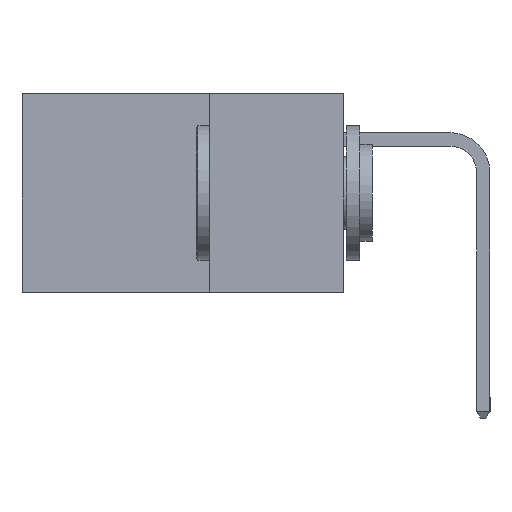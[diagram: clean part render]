
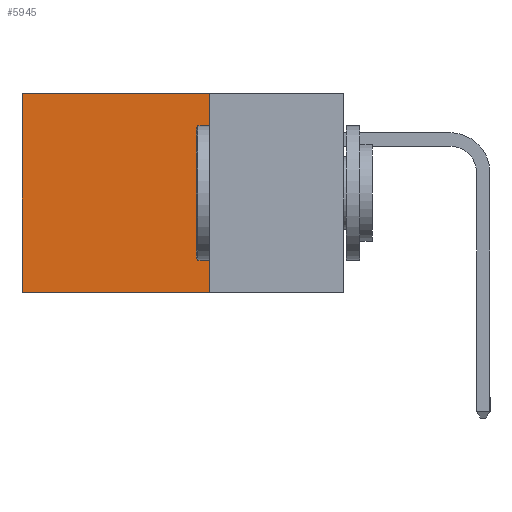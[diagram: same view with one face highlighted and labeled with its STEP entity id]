
A CAD part, left-side view. The second image highlights one B-rep face of the part: STEP entity #5945.
In plain terms, the highlighted planar face has unit normal (-1, 0, 0).
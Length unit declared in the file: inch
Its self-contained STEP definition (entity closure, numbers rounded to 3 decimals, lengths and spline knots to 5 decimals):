
#394 = VECTOR ( 'NONE', #13083, 39.37008 ) ;
#837 = VECTOR ( 'NONE', #13636, 39.37008 ) ;
#1482 = LINE ( 'NONE', #9746, #394 ) ;
#2814 = CARTESIAN_POINT ( 'NONE',  ( 0.2615, 0.25, -0.37 ) ) ;
#3259 = AXIS2_PLACEMENT_3D ( 'NONE', #7687, #7659, #7517 ) ;
#3355 = VERTEX_POINT ( 'NONE', #16010 ) ;
#3801 = LINE ( 'NONE', #19872, #16691 ) ;
#4559 = EDGE_CURVE ( 'NONE', #9637, #19219, #18807, .T. ) ;
#5437 = VECTOR ( 'NONE', #18161, 39.37008 ) ;
#5945 = ADVANCED_FACE ( 'NONE', ( #19355 ), #7998, .F. ) ;
#7511 = ORIENTED_EDGE ( 'NONE', *, *, #4559, .F. ) ;
#7517 = DIRECTION ( 'NONE',  ( 0., 0., -1. ) ) ;
#7659 = DIRECTION ( 'NONE',  ( 1., 0., 0. ) ) ;
#7687 = CARTESIAN_POINT ( 'NONE',  ( 0.2615, 0.25, -0.37 ) ) ;
#7998 = PLANE ( 'NONE',  #3259 ) ;
#8199 = DIRECTION ( 'NONE',  ( 0., 0., -1. ) ) ;
#9637 = VERTEX_POINT ( 'NONE', #2814 ) ;
#9746 = CARTESIAN_POINT ( 'NONE',  ( 0.2615, 0.25, 0. ) ) ;
#10069 = ORIENTED_EDGE ( 'NONE', *, *, #19935, .T. ) ;
#11668 = ORIENTED_EDGE ( 'NONE', *, *, #21297, .F. ) ;
#11946 = CARTESIAN_POINT ( 'NONE',  ( 0.2615, 0.25, -0.37 ) ) ;
#12007 = VERTEX_POINT ( 'NONE', #12186 ) ;
#12186 = CARTESIAN_POINT ( 'NONE',  ( 0.2615, 0.25, 0. ) ) ;
#13083 = DIRECTION ( 'NONE',  ( 0., 1., 0. ) ) ;
#13636 = DIRECTION ( 'NONE',  ( 0., 0., -1. ) ) ;
#14249 = LINE ( 'NONE', #11946, #837 ) ;
#15900 = CARTESIAN_POINT ( 'NONE',  ( 0.2615, 0.6, -0.37 ) ) ;
#16010 = CARTESIAN_POINT ( 'NONE',  ( 0.2615, 0.6, 0. ) ) ;
#16691 = VECTOR ( 'NONE', #8199, 39.37008 ) ;
#17437 = CARTESIAN_POINT ( 'NONE',  ( 0.2615, 0.25, -0.37 ) ) ;
#18161 = DIRECTION ( 'NONE',  ( 0., 1., 0. ) ) ;
#18313 = ORIENTED_EDGE ( 'NONE', *, *, #19986, .T. ) ;
#18807 = LINE ( 'NONE', #17437, #5437 ) ;
#19219 = VERTEX_POINT ( 'NONE', #15900 ) ;
#19355 = FACE_OUTER_BOUND ( 'NONE', #19636, .T. ) ;
#19636 = EDGE_LOOP ( 'NONE', ( #18313, #7511, #11668, #10069 ) ) ;
#19872 = CARTESIAN_POINT ( 'NONE',  ( 0.2615, 0.6, -0.37 ) ) ;
#19935 = EDGE_CURVE ( 'NONE', #12007, #3355, #1482, .T. ) ;
#19986 = EDGE_CURVE ( 'NONE', #3355, #19219, #3801, .T. ) ;
#21297 = EDGE_CURVE ( 'NONE', #12007, #9637, #14249, .T. ) ;
